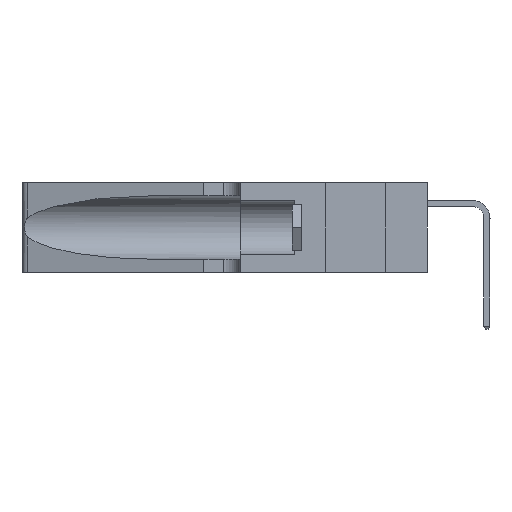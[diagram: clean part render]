
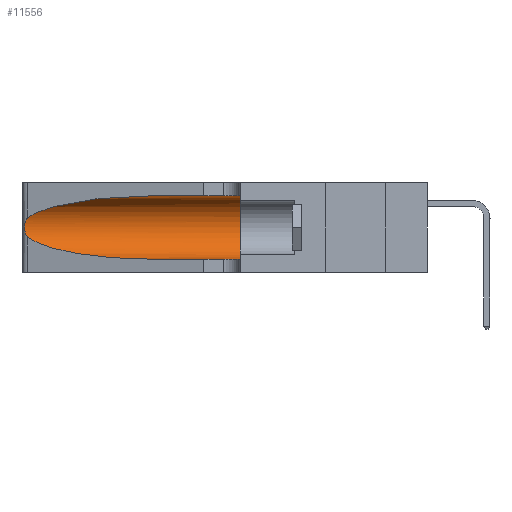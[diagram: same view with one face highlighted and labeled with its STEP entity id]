
A CAD part, left-side view. The second image highlights one B-rep face of the part: STEP entity #11556.
In plain terms, the highlighted cylindrical face has radius 3.308 mm (diameter 6.617 mm), a partial arc.
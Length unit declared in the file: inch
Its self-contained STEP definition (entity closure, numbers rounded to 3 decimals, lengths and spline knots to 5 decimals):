
#42 = CARTESIAN_POINT ( 'NONE',  ( 0.25487, 1.22718, 0.22369 ) ) ;
#766 = CARTESIAN_POINT ( 'NONE',  ( 0.26075, 1.23896, 0.19203 ) ) ;
#1169 = CARTESIAN_POINT ( 'NONE',  ( 0.25487, 1.22718, 0.22369 ) ) ;
#1225 = EDGE_CURVE ( 'NONE', #11424, #15731, #14883, .T. ) ;
#1810 = CARTESIAN_POINT ( 'NONE',  ( 0.25487, 1.22718, 0.22369 ) ) ;
#2264 = ORIENTED_EDGE ( 'NONE', *, *, #9084, .T. ) ;
#3246 = CYLINDRICAL_SURFACE ( 'NONE', #19305, 0.13025 ) ;
#3253 = ORIENTED_EDGE ( 'NONE', *, *, #25844, .T. ) ;
#3999 = CARTESIAN_POINT ( 'NONE',  ( 0.26017, 1.23833, 0.17102 ) ) ;
#4094 = VERTEX_POINT ( 'NONE', #17536 ) ;
#5627 =( BOUNDED_CURVE ( )  B_SPLINE_CURVE ( 3, ( #17722, #36867, #20954, #1810 ),
 .UNSPECIFIED., .F., .F. ) 
 B_SPLINE_CURVE_WITH_KNOTS ( ( 4, 4 ),
 ( 1.5708, 2.84003 ),
 .UNSPECIFIED. ) 
 CURVE ( )  GEOMETRIC_REPRESENTATION_ITEM ( )  RATIONAL_B_SPLINE_CURVE ( ( 1., 0.87, 0.87, 1. ) ) 
 REPRESENTATION_ITEM ( '' )  );
#5845 = LINE ( 'NONE', #8943, #14331 ) ;
#6343 = CARTESIAN_POINT ( 'NONE',  ( 0.1305, 0.72297, 0.05475 ) ) ;
#7220 = CARTESIAN_POINT ( 'NONE',  ( 0.25789, 1.23486, 0.15765 ) ) ;
#8943 = CARTESIAN_POINT ( 'NONE',  ( 0.1305, 1.61858, 0.31525 ) ) ;
#9084 = EDGE_CURVE ( 'NONE', #30747, #31731, #26416, .T. ) ;
#10431 = CARTESIAN_POINT ( 'NONE',  ( 0.25555, 1.22993, 0.14849 ) ) ;
#10549 =( BOUNDED_CURVE ( )  B_SPLINE_CURVE ( 3, ( #12628, #19014, #25464, #6343 ),
 .UNSPECIFIED., .F., .F. ) 
 B_SPLINE_CURVE_WITH_KNOTS ( ( 4, 4 ),
 ( 3.44316, 4.71239 ),
 .UNSPECIFIED. ) 
 CURVE ( )  GEOMETRIC_REPRESENTATION_ITEM ( )  RATIONAL_B_SPLINE_CURVE ( ( 1., 0.87, 0.87, 1. ) ) 
 REPRESENTATION_ITEM ( '' )  );
#11424 = VERTEX_POINT ( 'NONE', #1169 ) ;
#11556 = ADVANCED_FACE ( 'NONE', ( #28736 ), #3246, .F. ) ;
#12045 = CARTESIAN_POINT ( 'NONE',  ( 0.1305, 1.61858, 0.05475 ) ) ;
#12173 = DIRECTION ( 'NONE',  ( 0., -1., 0. ) ) ;
#12576 = CIRCLE ( 'NONE', #13840, 0.13025 ) ;
#12628 = CARTESIAN_POINT ( 'NONE',  ( 0.25487, 1.22718, 0.14631 ) ) ;
#13501 = CARTESIAN_POINT ( 'NONE',  ( 0.25555, 1.22994, 0.2215 ) ) ;
#13840 = AXIS2_PLACEMENT_3D ( 'NONE', #15432, #37783, #18624 ) ;
#14331 = VECTOR ( 'NONE', #12173, 39.37008 ) ;
#14594 = CARTESIAN_POINT ( 'NONE',  ( 0.1305, 1.61858, 0.185 ) ) ;
#14684 = ORIENTED_EDGE ( 'NONE', *, *, #41349, .F. ) ;
#14883 = B_SPLINE_CURVE_WITH_KNOTS ( 'NONE', 3,
 ( #42, #13501, #35831, #16669, #39065, #19922, #766, #23112, #3999, #26356, #7220, #29554, #10431, #32771 ),
 .UNSPECIFIED., .F., .F.,
 ( 4, 2, 2, 2, 2, 2, 4 ),
 ( 0., 0.00027, 0.00053, 0.00107, 0.0016, 0.00187, 0.00214 ),
 .UNSPECIFIED. ) ;
#15392 = ORIENTED_EDGE ( 'NONE', *, *, #1225, .T. ) ;
#15432 = CARTESIAN_POINT ( 'NONE',  ( 0.1305, 0.35, 0.185 ) ) ;
#15477 = EDGE_CURVE ( 'NONE', #35346, #4094, #5845, .T. ) ;
#15731 = VERTEX_POINT ( 'NONE', #38957 ) ;
#16669 = CARTESIAN_POINT ( 'NONE',  ( 0.25787, 1.23484, 0.2124 ) ) ;
#17536 = CARTESIAN_POINT ( 'NONE',  ( 0.1305, 0.35, 0.31525 ) ) ;
#17722 = CARTESIAN_POINT ( 'NONE',  ( 0.1305, 0.72297, 0.31525 ) ) ;
#18154 = EDGE_LOOP ( 'NONE', ( #3253, #15392, #37226, #2264, #14684, #40940 ) ) ;
#18624 = DIRECTION ( 'NONE',  ( 0., 0., 1. ) ) ;
#19014 = CARTESIAN_POINT ( 'NONE',  ( 0.2373, 1.15595, 0.08982 ) ) ;
#19305 = AXIS2_PLACEMENT_3D ( 'NONE', #14594, #36935, #30528 ) ;
#19922 = CARTESIAN_POINT ( 'NONE',  ( 0.26018, 1.23835, 0.19895 ) ) ;
#20954 = CARTESIAN_POINT ( 'NONE',  ( 0.2373, 1.15595, 0.28018 ) ) ;
#21422 = EDGE_CURVE ( 'NONE', #15731, #30747, #10549, .T. ) ;
#23112 = CARTESIAN_POINT ( 'NONE',  ( 0.26075, 1.23896, 0.178 ) ) ;
#25464 = CARTESIAN_POINT ( 'NONE',  ( 0.18966, 0.96281, 0.05475 ) ) ;
#25844 = EDGE_CURVE ( 'NONE', #35346, #11424, #5627, .T. ) ;
#26356 = CARTESIAN_POINT ( 'NONE',  ( 0.25856, 1.23593, 0.16098 ) ) ;
#26416 = LINE ( 'NONE', #12045, #36895 ) ;
#26615 = CARTESIAN_POINT ( 'NONE',  ( 0.1305, 0.72297, 0.31525 ) ) ;
#28736 = FACE_OUTER_BOUND ( 'NONE', #18154, .T. ) ;
#29554 = CARTESIAN_POINT ( 'NONE',  ( 0.25639, 1.23186, 0.15144 ) ) ;
#30528 = DIRECTION ( 'NONE',  ( 0., 0., -1. ) ) ;
#30726 = CARTESIAN_POINT ( 'NONE',  ( 0.1305, 0.72297, 0.05475 ) ) ;
#30747 = VERTEX_POINT ( 'NONE', #30726 ) ;
#31731 = VERTEX_POINT ( 'NONE', #33823 ) ;
#32771 = CARTESIAN_POINT ( 'NONE',  ( 0.25487, 1.22718, 0.14631 ) ) ;
#33823 = CARTESIAN_POINT ( 'NONE',  ( 0.1305, 0.35, 0.05475 ) ) ;
#34395 = DIRECTION ( 'NONE',  ( 0., -1., 0. ) ) ;
#35346 = VERTEX_POINT ( 'NONE', #26615 ) ;
#35831 = CARTESIAN_POINT ( 'NONE',  ( 0.25639, 1.23184, 0.21858 ) ) ;
#36867 = CARTESIAN_POINT ( 'NONE',  ( 0.18966, 0.96281, 0.31525 ) ) ;
#36895 = VECTOR ( 'NONE', #34395, 39.37008 ) ;
#36935 = DIRECTION ( 'NONE',  ( 0., -1., 0. ) ) ;
#37226 = ORIENTED_EDGE ( 'NONE', *, *, #21422, .T. ) ;
#37783 = DIRECTION ( 'NONE',  ( 0., 1., 0. ) ) ;
#38957 = CARTESIAN_POINT ( 'NONE',  ( 0.25487, 1.22718, 0.14631 ) ) ;
#39065 = CARTESIAN_POINT ( 'NONE',  ( 0.25854, 1.2359, 0.20912 ) ) ;
#40940 = ORIENTED_EDGE ( 'NONE', *, *, #15477, .F. ) ;
#41349 = EDGE_CURVE ( 'NONE', #4094, #31731, #12576, .T. ) ;
